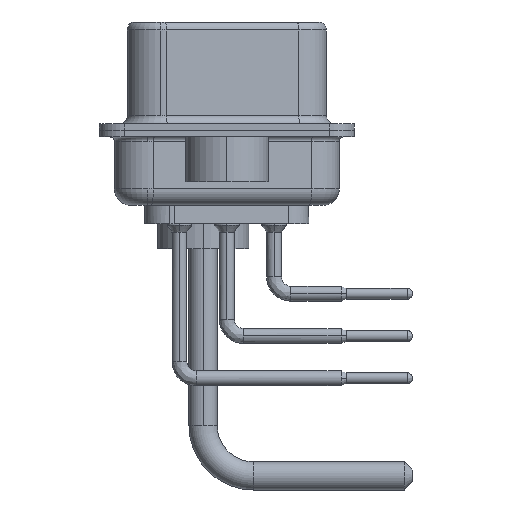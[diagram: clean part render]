
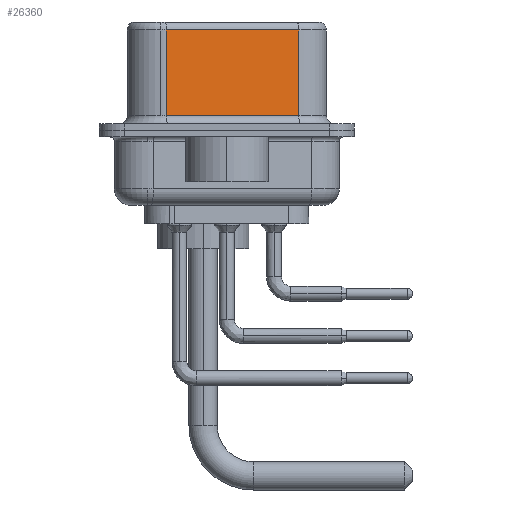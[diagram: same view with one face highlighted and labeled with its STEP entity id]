
A CAD part, left-side view. The second image highlights one B-rep face of the part: STEP entity #26360.
In plain terms, the highlighted planar face has unit normal (-0.985, -0.174, 0).
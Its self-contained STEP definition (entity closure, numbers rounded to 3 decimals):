
#208 = LINE ( 'NONE', #11402, #18286 ) ;
#1352 = CARTESIAN_POINT ( 'NONE',  ( 3.73, 3.628, 6.02 ) ) ;
#2619 = DIRECTION ( 'NONE',  ( -0.174, 0.985, 0. ) ) ;
#3057 = VECTOR ( 'NONE', #4992, 1000. ) ;
#4992 = DIRECTION ( 'NONE',  ( 0., 0., -1. ) ) ;
#5033 = FACE_OUTER_BOUND ( 'NONE', #36213, .T. ) ;
#5726 = CARTESIAN_POINT ( 'NONE',  ( 5.132, -4.322, 6.52 ) ) ;
#6722 = VERTEX_POINT ( 'NONE', #1352 ) ;
#7280 = VERTEX_POINT ( 'NONE', #16693 ) ;
#7395 = CARTESIAN_POINT ( 'NONE',  ( 5.132, -4.322, 0.9 ) ) ;
#8261 = EDGE_CURVE ( 'NONE', #6722, #13766, #29033, .T. ) ;
#9738 = CARTESIAN_POINT ( 'NONE',  ( 3.73, 3.628, 6.52 ) ) ;
#10701 = ORIENTED_EDGE ( 'NONE', *, *, #32444, .T. ) ;
#11387 = AXIS2_PLACEMENT_3D ( 'NONE', #16557, #16385, #2619 ) ;
#11402 = CARTESIAN_POINT ( 'NONE',  ( 5.132, -4.322, 6.02 ) ) ;
#12515 = ORIENTED_EDGE ( 'NONE', *, *, #32665, .T. ) ;
#12725 = LINE ( 'NONE', #7395, #22401 ) ;
#13766 = VERTEX_POINT ( 'NONE', #21768 ) ;
#14206 = ORIENTED_EDGE ( 'NONE', *, *, #8261, .T. ) ;
#16385 = DIRECTION ( 'NONE',  ( 0.985, 0.174, 0. ) ) ;
#16557 = CARTESIAN_POINT ( 'NONE',  ( 5.132, -4.322, 6.52 ) ) ;
#16693 = CARTESIAN_POINT ( 'NONE',  ( 5.132, -4.322, 6.02 ) ) ;
#18286 = VECTOR ( 'NONE', #22786, 1000. ) ;
#19499 = PLANE ( 'NONE',  #11387 ) ;
#20513 = DIRECTION ( 'NONE',  ( 0., 0., -1. ) ) ;
#21629 = EDGE_CURVE ( 'NONE', #7280, #32009, #36187, .T. ) ;
#21768 = CARTESIAN_POINT ( 'NONE',  ( 3.73, 3.628, 0.9 ) ) ;
#22401 = VECTOR ( 'NONE', #23927, 1000. ) ;
#22786 = DIRECTION ( 'NONE',  ( -0.174, 0.985, 0. ) ) ;
#23927 = DIRECTION ( 'NONE',  ( 0.174, -0.985, 0. ) ) ;
#24091 = VECTOR ( 'NONE', #20513, 1000. ) ;
#26360 = ADVANCED_FACE ( 'NONE', ( #5033 ), #19499, .F. ) ;
#27585 = ORIENTED_EDGE ( 'NONE', *, *, #21629, .F. ) ;
#27802 = CARTESIAN_POINT ( 'NONE',  ( 5.132, -4.322, 0.9 ) ) ;
#29033 = LINE ( 'NONE', #9738, #3057 ) ;
#32009 = VERTEX_POINT ( 'NONE', #27802 ) ;
#32444 = EDGE_CURVE ( 'NONE', #13766, #32009, #12725, .T. ) ;
#32665 = EDGE_CURVE ( 'NONE', #7280, #6722, #208, .T. ) ;
#36187 = LINE ( 'NONE', #5726, #24091 ) ;
#36213 = EDGE_LOOP ( 'NONE', ( #27585, #12515, #14206, #10701 ) ) ;
